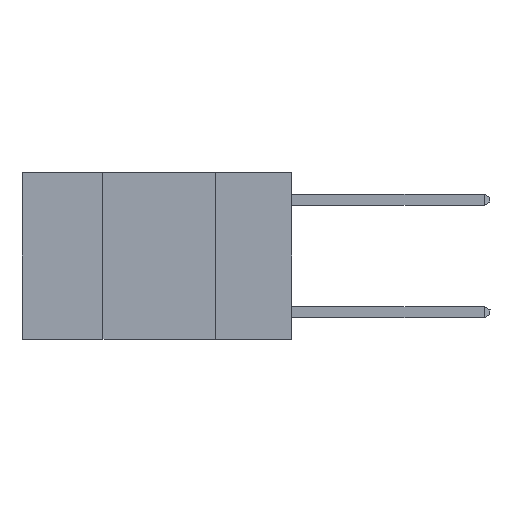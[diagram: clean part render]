
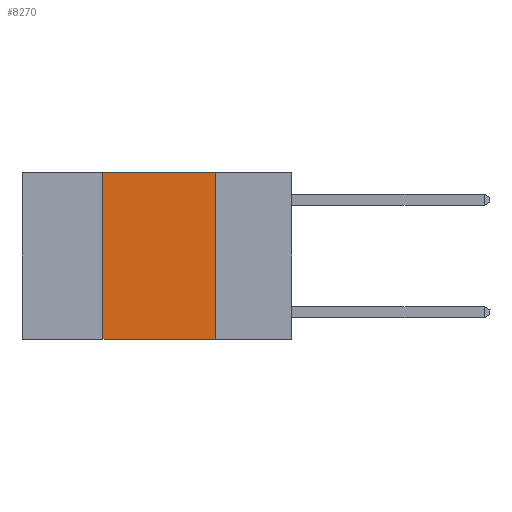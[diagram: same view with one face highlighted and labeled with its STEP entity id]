
A CAD part, left-side view. The second image highlights one B-rep face of the part: STEP entity #8270.
In plain terms, the highlighted planar face has unit normal (-1, 0, 0).
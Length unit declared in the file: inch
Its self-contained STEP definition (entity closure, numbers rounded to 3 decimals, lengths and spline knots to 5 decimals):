
#175 = CARTESIAN_POINT ( 'NONE',  ( 0., 0.6, -0.37 ) ) ;
#1008 = VECTOR ( 'NONE', #16358, 39.37008 ) ;
#1246 = VECTOR ( 'NONE', #6817, 39.37008 ) ;
#1688 = LINE ( 'NONE', #2696, #1246 ) ;
#2393 = PLANE ( 'NONE',  #17031 ) ;
#2461 = DIRECTION ( 'NONE',  ( 0., 0., -1. ) ) ;
#2696 = CARTESIAN_POINT ( 'NONE',  ( 0., 0.6, 0. ) ) ;
#2923 = VECTOR ( 'NONE', #7348, 39.37008 ) ;
#4453 = FACE_OUTER_BOUND ( 'NONE', #14690, .T. ) ;
#4454 = VERTEX_POINT ( 'NONE', #7178 ) ;
#6574 = LINE ( 'NONE', #16814, #2923 ) ;
#6817 = DIRECTION ( 'NONE',  ( 0., -1., 0. ) ) ;
#7178 = CARTESIAN_POINT ( 'NONE',  ( 0., 0.17, 0. ) ) ;
#7348 = DIRECTION ( 'NONE',  ( 0., 0., 1. ) ) ;
#8227 = CARTESIAN_POINT ( 'NONE',  ( 0., 0.17, 0. ) ) ;
#8270 = ADVANCED_FACE ( 'NONE', ( #4453 ), #2393, .F. ) ;
#8369 = EDGE_CURVE ( 'NONE', #16071, #4454, #1688, .T. ) ;
#9028 = CARTESIAN_POINT ( 'NONE',  ( 0., 0.42, 0. ) ) ;
#9152 = EDGE_CURVE ( 'NONE', #4454, #17046, #11201, .T. ) ;
#9499 = ORIENTED_EDGE ( 'NONE', *, *, #9152, .F. ) ;
#9732 = CARTESIAN_POINT ( 'NONE',  ( 0., 0.17, -0.37 ) ) ;
#9965 = VECTOR ( 'NONE', #13939, 39.37008 ) ;
#10739 = DIRECTION ( 'NONE',  ( 1., 0., 0. ) ) ;
#11201 = LINE ( 'NONE', #8227, #1008 ) ;
#11298 = CARTESIAN_POINT ( 'NONE',  ( 0., 0.42, -0.37 ) ) ;
#12712 = ORIENTED_EDGE ( 'NONE', *, *, #14152, .T. ) ;
#12836 = VERTEX_POINT ( 'NONE', #11298 ) ;
#13939 = DIRECTION ( 'NONE',  ( 0., -1., 0. ) ) ;
#14152 = EDGE_CURVE ( 'NONE', #12836, #17046, #17122, .T. ) ;
#14690 = EDGE_LOOP ( 'NONE', ( #9499, #17094, #15200, #12712 ) ) ;
#15200 = ORIENTED_EDGE ( 'NONE', *, *, #16619, .F. ) ;
#16066 = CARTESIAN_POINT ( 'NONE',  ( 0., 0.6, 0. ) ) ;
#16071 = VERTEX_POINT ( 'NONE', #9028 ) ;
#16358 = DIRECTION ( 'NONE',  ( 0., 0., -1. ) ) ;
#16619 = EDGE_CURVE ( 'NONE', #12836, #16071, #6574, .T. ) ;
#16814 = CARTESIAN_POINT ( 'NONE',  ( 0., 0.42, 0. ) ) ;
#17031 = AXIS2_PLACEMENT_3D ( 'NONE', #16066, #10739, #2461 ) ;
#17046 = VERTEX_POINT ( 'NONE', #9732 ) ;
#17094 = ORIENTED_EDGE ( 'NONE', *, *, #8369, .F. ) ;
#17122 = LINE ( 'NONE', #175, #9965 ) ;
